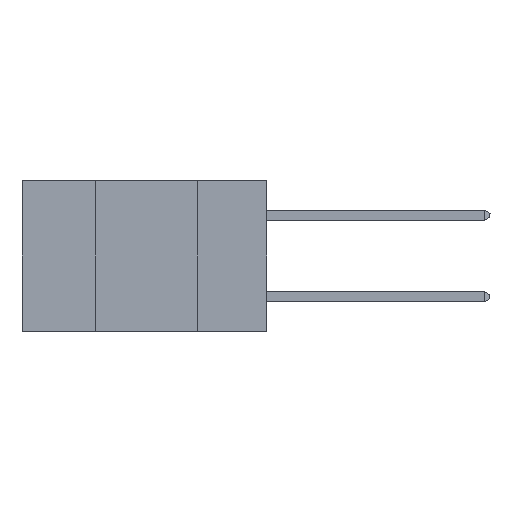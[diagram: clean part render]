
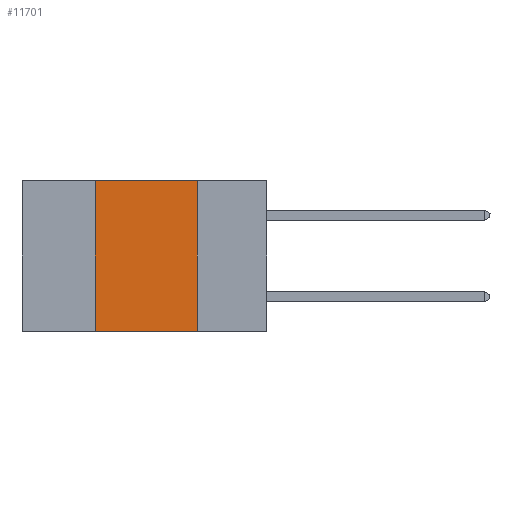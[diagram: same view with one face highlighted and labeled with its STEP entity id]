
A CAD part, left-side view. The second image highlights one B-rep face of the part: STEP entity #11701.
In plain terms, the highlighted planar face has unit normal (-1, 0, 0).
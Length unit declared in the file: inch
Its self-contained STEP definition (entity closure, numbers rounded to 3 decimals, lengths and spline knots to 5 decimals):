
#522 = CARTESIAN_POINT ( 'NONE',  ( 0., 0.17, 0. ) ) ;
#1825 = DIRECTION ( 'NONE',  ( 0., 0., 1. ) ) ;
#2154 = EDGE_CURVE ( 'NONE', #14784, #14587, #3706, .T. ) ;
#2451 = EDGE_CURVE ( 'NONE', #14784, #13965, #13292, .T. ) ;
#2476 = CARTESIAN_POINT ( 'NONE',  ( 0., 0.6, 0. ) ) ;
#2530 = VECTOR ( 'NONE', #17449, 39.37008 ) ;
#3706 = LINE ( 'NONE', #24406, #5750 ) ;
#3752 = ORIENTED_EDGE ( 'NONE', *, *, #2451, .T. ) ;
#3793 = CARTESIAN_POINT ( 'NONE',  ( 0., 0.6, 0. ) ) ;
#4460 = ORIENTED_EDGE ( 'NONE', *, *, #14087, .F. ) ;
#4507 = CARTESIAN_POINT ( 'NONE',  ( 0., 0.42, 0. ) ) ;
#5511 = AXIS2_PLACEMENT_3D ( 'NONE', #2476, #12369, #12227 ) ;
#5750 = VECTOR ( 'NONE', #1825, 39.37008 ) ;
#6486 = FACE_OUTER_BOUND ( 'NONE', #16171, .T. ) ;
#6754 = PLANE ( 'NONE',  #5511 ) ;
#9638 = VERTEX_POINT ( 'NONE', #11471 ) ;
#9753 = CARTESIAN_POINT ( 'NONE',  ( 0., 0.17, -0.37 ) ) ;
#11471 = CARTESIAN_POINT ( 'NONE',  ( 0., 0.17, 0. ) ) ;
#11701 = ADVANCED_FACE ( 'NONE', ( #6486 ), #6754, .F. ) ;
#12022 = VECTOR ( 'NONE', #24844, 39.37008 ) ;
#12227 = DIRECTION ( 'NONE',  ( 0., 0., -1. ) ) ;
#12369 = DIRECTION ( 'NONE',  ( 1., 0., 0. ) ) ;
#12420 = LINE ( 'NONE', #522, #12022 ) ;
#13292 = LINE ( 'NONE', #25332, #2530 ) ;
#13855 = ORIENTED_EDGE ( 'NONE', *, *, #2154, .F. ) ;
#13965 = VERTEX_POINT ( 'NONE', #9753 ) ;
#14087 = EDGE_CURVE ( 'NONE', #9638, #13965, #12420, .T. ) ;
#14338 = LINE ( 'NONE', #3793, #18266 ) ;
#14587 = VERTEX_POINT ( 'NONE', #4507 ) ;
#14784 = VERTEX_POINT ( 'NONE', #19600 ) ;
#16171 = EDGE_LOOP ( 'NONE', ( #4460, #20376, #13855, #3752 ) ) ;
#17449 = DIRECTION ( 'NONE',  ( 0., -1., 0. ) ) ;
#18266 = VECTOR ( 'NONE', #22491, 39.37008 ) ;
#19600 = CARTESIAN_POINT ( 'NONE',  ( 0., 0.42, -0.37 ) ) ;
#20376 = ORIENTED_EDGE ( 'NONE', *, *, #21867, .F. ) ;
#21867 = EDGE_CURVE ( 'NONE', #14587, #9638, #14338, .T. ) ;
#22491 = DIRECTION ( 'NONE',  ( 0., -1., 0. ) ) ;
#24406 = CARTESIAN_POINT ( 'NONE',  ( 0., 0.42, 0. ) ) ;
#24844 = DIRECTION ( 'NONE',  ( 0., 0., -1. ) ) ;
#25332 = CARTESIAN_POINT ( 'NONE',  ( 0., 0.6, -0.37 ) ) ;
